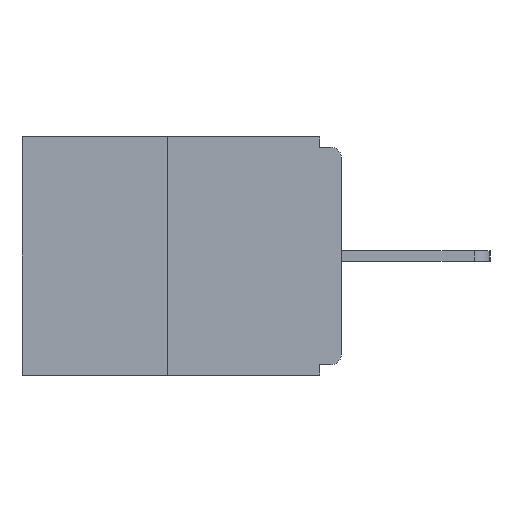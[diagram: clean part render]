
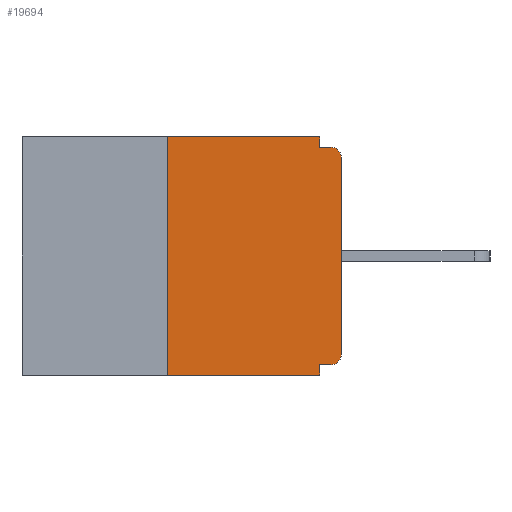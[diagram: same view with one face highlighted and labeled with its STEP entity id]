
A CAD part, left-side view. The second image highlights one B-rep face of the part: STEP entity #19694.
In plain terms, the highlighted planar face has unit normal (-1, 0, 0).
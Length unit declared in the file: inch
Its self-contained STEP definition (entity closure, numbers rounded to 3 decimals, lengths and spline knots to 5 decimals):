
#107 = EDGE_CURVE ( 'NONE', #20745, #20826, #13369, .T. ) ;
#1226 = ORIENTED_EDGE ( 'NONE', *, *, #7400, .F. ) ;
#1395 = ORIENTED_EDGE ( 'NONE', *, *, #107, .F. ) ;
#1439 = ORIENTED_EDGE ( 'NONE', *, *, #3618, .T. ) ;
#1550 = ORIENTED_EDGE ( 'NONE', *, *, #20362, .F. ) ;
#1678 = ORIENTED_EDGE ( 'NONE', *, *, #2929, .F. ) ;
#1846 = ORIENTED_EDGE ( 'NONE', *, *, #3753, .T. ) ;
#2065 = ORIENTED_EDGE ( 'NONE', *, *, #22176, .T. ) ;
#2140 = ORIENTED_EDGE ( 'NONE', *, *, #14564, .T. ) ;
#2329 = ORIENTED_EDGE ( 'NONE', *, *, #20783, .F. ) ;
#2526 = FACE_OUTER_BOUND ( 'NONE', #9749, .T. ) ;
#2543 = ORIENTED_EDGE ( 'NONE', *, *, #12565, .F. ) ;
#2768 = CARTESIAN_POINT ( 'NONE',  ( 0., 0.015, -0.03 ) ) ;
#2793 = CARTESIAN_POINT ( 'NONE',  ( 0., 0.031, -0.343 ) ) ;
#2929 = EDGE_CURVE ( 'NONE', #12892, #21386, #9157, .T. ) ;
#3173 = DIRECTION ( 'NONE',  ( 0., 0., 1. ) ) ;
#3337 = CARTESIAN_POINT ( 'NONE',  ( 0., 0.015, -0.328 ) ) ;
#3488 = VECTOR ( 'NONE', #8880, 39.37008 ) ;
#3560 = VECTOR ( 'NONE', #13917, 39.37008 ) ;
#3618 = EDGE_CURVE ( 'NONE', #20745, #12847, #8822, .T. ) ;
#3753 = EDGE_CURVE ( 'NONE', #12892, #4947, #19769, .T. ) ;
#3901 = CARTESIAN_POINT ( 'NONE',  ( 0., 0.031, -0.015 ) ) ;
#4072 = VECTOR ( 'NONE', #3173, 39.37008 ) ;
#4149 = LINE ( 'NONE', #2793, #3560 ) ;
#4195 = VECTOR ( 'NONE', #10588, 39.37008 ) ;
#4221 = CARTESIAN_POINT ( 'NONE',  ( 0., 0.25, 0. ) ) ;
#4441 = CARTESIAN_POINT ( 'NONE',  ( 0., 0.031, -0.328 ) ) ;
#4545 = LINE ( 'NONE', #10036, #22516 ) ;
#4666 = DIRECTION ( 'NONE',  ( 0., 0., -1. ) ) ;
#4947 = VERTEX_POINT ( 'NONE', #12627 ) ;
#6009 = CARTESIAN_POINT ( 'NONE',  ( 0., 0.46, 0. ) ) ;
#6206 = CARTESIAN_POINT ( 'NONE',  ( 0., 0.031, 0. ) ) ;
#6990 = CARTESIAN_POINT ( 'NONE',  ( 0., 0., 0. ) ) ;
#7017 = CARTESIAN_POINT ( 'NONE',  ( 0., 0.031, -0.343 ) ) ;
#7315 = DIRECTION ( 'NONE',  ( 0., -1., 0. ) ) ;
#7400 = EDGE_CURVE ( 'NONE', #20826, #8568, #4545, .T. ) ;
#7679 = CARTESIAN_POINT ( 'NONE',  ( 0., 0.25, -0.343 ) ) ;
#7871 = CARTESIAN_POINT ( 'NONE',  ( 0., 0.46, -0.343 ) ) ;
#7873 = DIRECTION ( 'NONE',  ( 1., 0., 0. ) ) ;
#8043 = CARTESIAN_POINT ( 'NONE',  ( 0., 0.25, 0. ) ) ;
#8080 = DIRECTION ( 'NONE',  ( 0., 0., -1. ) ) ;
#8568 = VERTEX_POINT ( 'NONE', #11447 ) ;
#8822 = LINE ( 'NONE', #7871, #17902 ) ;
#8880 = DIRECTION ( 'NONE',  ( 0., 0., 1. ) ) ;
#8955 = LINE ( 'NONE', #6206, #14420 ) ;
#9157 = LINE ( 'NONE', #10212, #4195 ) ;
#9554 = VERTEX_POINT ( 'NONE', #21443 ) ;
#9749 = EDGE_LOOP ( 'NONE', ( #1226, #1395, #1439, #1550, #1678, #1846, #2065, #2140, #2329, #2543 ) ) ;
#10036 = CARTESIAN_POINT ( 'NONE',  ( 0., 0.46, 0. ) ) ;
#10212 = CARTESIAN_POINT ( 'NONE',  ( 0., 0., -0.328 ) ) ;
#10588 = DIRECTION ( 'NONE',  ( 0., 1., 0. ) ) ;
#10912 = DIRECTION ( 'NONE',  ( 0., 0., -1. ) ) ;
#11447 = CARTESIAN_POINT ( 'NONE',  ( 0., 0.031, 0. ) ) ;
#11656 = VERTEX_POINT ( 'NONE', #3901 ) ;
#11910 = DIRECTION ( 'NONE',  ( 0., -1., 0. ) ) ;
#12286 = LINE ( 'NONE', #20420, #21079 ) ;
#12565 = EDGE_CURVE ( 'NONE', #8568, #11656, #8955, .T. ) ;
#12627 = CARTESIAN_POINT ( 'NONE',  ( 0., 0., -0.313 ) ) ;
#12847 = VERTEX_POINT ( 'NONE', #7017 ) ;
#12892 = VERTEX_POINT ( 'NONE', #3337 ) ;
#13369 = LINE ( 'NONE', #8043, #4072 ) ;
#13885 = AXIS2_PLACEMENT_3D ( 'NONE', #2768, #15706, #4666 ) ;
#13917 = DIRECTION ( 'NONE',  ( 0., 0., -1. ) ) ;
#14420 = VECTOR ( 'NONE', #8080, 39.37008 ) ;
#14564 = EDGE_CURVE ( 'NONE', #9554, #17702, #23061, .T. ) ;
#15096 = CARTESIAN_POINT ( 'NONE',  ( 0., 0.015, -0.015 ) ) ;
#15161 = DIRECTION ( 'NONE',  ( 0., -1., 0. ) ) ;
#15706 = DIRECTION ( 'NONE',  ( -1., 0., 0. ) ) ;
#15847 = DIRECTION ( 'NONE',  ( -1., 0., 0. ) ) ;
#15849 = CARTESIAN_POINT ( 'NONE',  ( 0., 0.015, -0.313 ) ) ;
#16998 = PLANE ( 'NONE',  #22710 ) ;
#17702 = VERTEX_POINT ( 'NONE', #15096 ) ;
#17902 = VECTOR ( 'NONE', #7315, 39.37008 ) ;
#18108 = LINE ( 'NONE', #6990, #3488 ) ;
#19694 = ADVANCED_FACE ( 'NONE', ( #2526 ), #16998, .F. ) ;
#19769 = CIRCLE ( 'NONE', #20974, 0.015 ) ;
#20362 = EDGE_CURVE ( 'NONE', #21386, #12847, #4149, .T. ) ;
#20420 = CARTESIAN_POINT ( 'NONE',  ( 0., 0., -0.015 ) ) ;
#20464 = DIRECTION ( 'NONE',  ( 0., 0., -1. ) ) ;
#20745 = VERTEX_POINT ( 'NONE', #7679 ) ;
#20783 = EDGE_CURVE ( 'NONE', #11656, #17702, #12286, .T. ) ;
#20826 = VERTEX_POINT ( 'NONE', #4221 ) ;
#20974 = AXIS2_PLACEMENT_3D ( 'NONE', #15849, #15847, #10912 ) ;
#21079 = VECTOR ( 'NONE', #15161, 39.37008 ) ;
#21386 = VERTEX_POINT ( 'NONE', #4441 ) ;
#21443 = CARTESIAN_POINT ( 'NONE',  ( 0., 0., -0.03 ) ) ;
#22176 = EDGE_CURVE ( 'NONE', #4947, #9554, #18108, .T. ) ;
#22516 = VECTOR ( 'NONE', #11910, 39.37008 ) ;
#22710 = AXIS2_PLACEMENT_3D ( 'NONE', #6009, #7873, #20464 ) ;
#23061 = CIRCLE ( 'NONE', #13885, 0.015 ) ;
